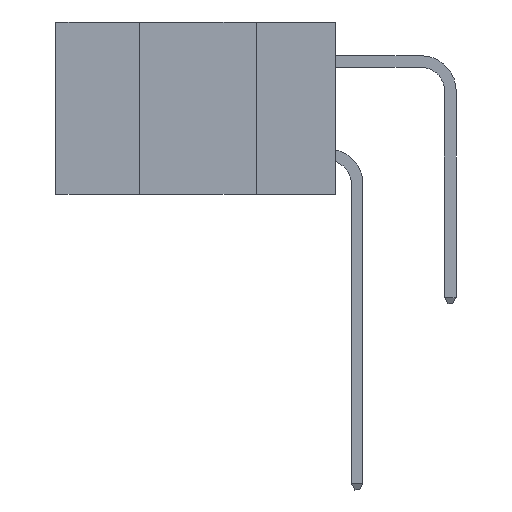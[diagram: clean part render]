
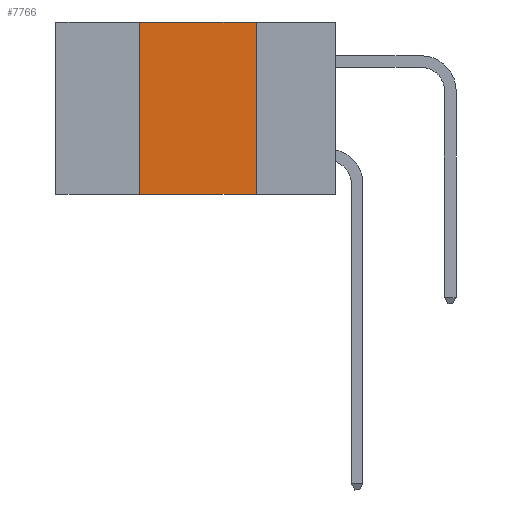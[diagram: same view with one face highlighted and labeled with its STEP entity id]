
A CAD part, left-side view. The second image highlights one B-rep face of the part: STEP entity #7766.
In plain terms, the highlighted planar face has unit normal (-1, 0, 0).
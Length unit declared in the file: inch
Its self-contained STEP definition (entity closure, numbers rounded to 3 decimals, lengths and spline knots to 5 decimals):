
#48 = ORIENTED_EDGE ( 'NONE', *, *, #11941, .F. ) ;
#187 = VECTOR ( 'NONE', #4155, 39.37008 ) ;
#263 = EDGE_CURVE ( 'NONE', #2514, #5902, #12233, .T. ) ;
#417 = LINE ( 'NONE', #5719, #9913 ) ;
#762 = VECTOR ( 'NONE', #1052, 39.37008 ) ;
#1052 = DIRECTION ( 'NONE',  ( 0., 0., -1. ) ) ;
#2514 = VERTEX_POINT ( 'NONE', #12694 ) ;
#2792 = CARTESIAN_POINT ( 'NONE',  ( 0., 0.17, -0.37 ) ) ;
#4000 = CARTESIAN_POINT ( 'NONE',  ( 0., 0.6, 0. ) ) ;
#4155 = DIRECTION ( 'NONE',  ( 0., -1., 0. ) ) ;
#4844 = VERTEX_POINT ( 'NONE', #9524 ) ;
#4968 = LINE ( 'NONE', #7253, #762 ) ;
#5225 = DIRECTION ( 'NONE',  ( 0., 0., -1. ) ) ;
#5719 = CARTESIAN_POINT ( 'NONE',  ( 0., 0.6, 0. ) ) ;
#5902 = VERTEX_POINT ( 'NONE', #8686 ) ;
#5935 = DIRECTION ( 'NONE',  ( 0., 0., 1. ) ) ;
#7253 = CARTESIAN_POINT ( 'NONE',  ( 0., 0.17, 0. ) ) ;
#7429 = VECTOR ( 'NONE', #5935, 39.37008 ) ;
#7605 = VERTEX_POINT ( 'NONE', #2792 ) ;
#7766 = ADVANCED_FACE ( 'NONE', ( #13247 ), #8225, .F. ) ;
#8225 = PLANE ( 'NONE',  #9098 ) ;
#8686 = CARTESIAN_POINT ( 'NONE',  ( 0., 0.42, 0. ) ) ;
#8789 = ORIENTED_EDGE ( 'NONE', *, *, #9629, .T. ) ;
#9098 = AXIS2_PLACEMENT_3D ( 'NONE', #4000, #11381, #5225 ) ;
#9524 = CARTESIAN_POINT ( 'NONE',  ( 0., 0.17, 0. ) ) ;
#9629 = EDGE_CURVE ( 'NONE', #2514, #7605, #12430, .T. ) ;
#9913 = VECTOR ( 'NONE', #9970, 39.37008 ) ;
#9970 = DIRECTION ( 'NONE',  ( 0., -1., 0. ) ) ;
#11344 = CARTESIAN_POINT ( 'NONE',  ( 0., 0.6, -0.37 ) ) ;
#11381 = DIRECTION ( 'NONE',  ( 1., 0., 0. ) ) ;
#11668 = EDGE_LOOP ( 'NONE', ( #48, #13056, #11826, #8789 ) ) ;
#11826 = ORIENTED_EDGE ( 'NONE', *, *, #263, .F. ) ;
#11941 = EDGE_CURVE ( 'NONE', #4844, #7605, #4968, .T. ) ;
#12087 = CARTESIAN_POINT ( 'NONE',  ( 0., 0.42, 0. ) ) ;
#12144 = EDGE_CURVE ( 'NONE', #5902, #4844, #417, .T. ) ;
#12233 = LINE ( 'NONE', #12087, #7429 ) ;
#12430 = LINE ( 'NONE', #11344, #187 ) ;
#12694 = CARTESIAN_POINT ( 'NONE',  ( 0., 0.42, -0.37 ) ) ;
#13056 = ORIENTED_EDGE ( 'NONE', *, *, #12144, .F. ) ;
#13247 = FACE_OUTER_BOUND ( 'NONE', #11668, .T. ) ;
